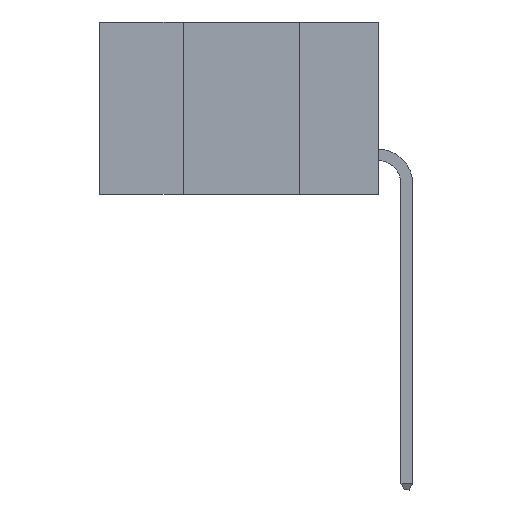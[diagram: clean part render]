
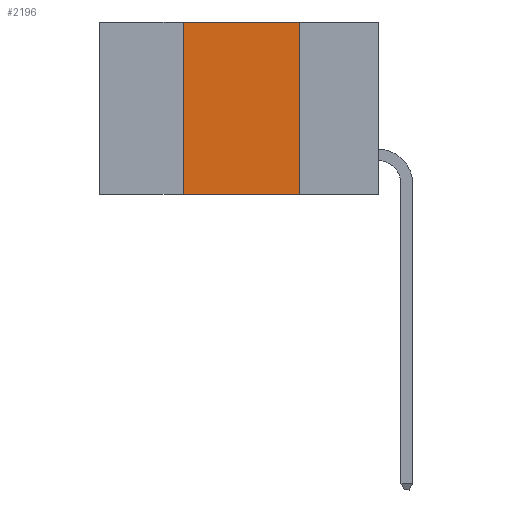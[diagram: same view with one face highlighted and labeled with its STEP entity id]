
A CAD part, left-side view. The second image highlights one B-rep face of the part: STEP entity #2196.
In plain terms, the highlighted planar face has unit normal (-1, 0, 0).
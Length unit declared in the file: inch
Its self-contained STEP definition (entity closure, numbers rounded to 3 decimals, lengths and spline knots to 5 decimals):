
#313 = ORIENTED_EDGE ( 'NONE', *, *, #7847, .T. ) ;
#606 = ORIENTED_EDGE ( 'NONE', *, *, #3129, .F. ) ;
#937 = VECTOR ( 'NONE', #29486, 39.37008 ) ;
#1096 = DIRECTION ( 'NONE',  ( 0., -1., 0. ) ) ;
#1657 = VERTEX_POINT ( 'NONE', #4652 ) ;
#1899 = CARTESIAN_POINT ( 'NONE',  ( 0., 0.6, 0. ) ) ;
#2196 = ADVANCED_FACE ( 'NONE', ( #18134 ), #19116, .F. ) ;
#2372 = LINE ( 'NONE', #12131, #5848 ) ;
#2737 = VERTEX_POINT ( 'NONE', #16178 ) ;
#3129 = EDGE_CURVE ( 'NONE', #22476, #1657, #28222, .T. ) ;
#4652 = CARTESIAN_POINT ( 'NONE',  ( 0., 0.17, 0. ) ) ;
#5111 = DIRECTION ( 'NONE',  ( 0., -1., 0. ) ) ;
#5848 = VECTOR ( 'NONE', #5111, 39.37008 ) ;
#6879 = DIRECTION ( 'NONE',  ( 1., 0., 0. ) ) ;
#7847 = EDGE_CURVE ( 'NONE', #23846, #2737, #2372, .T. ) ;
#7997 = VECTOR ( 'NONE', #1096, 39.37008 ) ;
#10301 = ORIENTED_EDGE ( 'NONE', *, *, #19878, .F. ) ;
#12131 = CARTESIAN_POINT ( 'NONE',  ( 0., 0.6, -0.37 ) ) ;
#12479 = DIRECTION ( 'NONE',  ( 0., 0., 1. ) ) ;
#12748 = LINE ( 'NONE', #29764, #24333 ) ;
#13990 = ORIENTED_EDGE ( 'NONE', *, *, #15978, .F. ) ;
#15978 = EDGE_CURVE ( 'NONE', #1657, #2737, #28776, .T. ) ;
#16178 = CARTESIAN_POINT ( 'NONE',  ( 0., 0.17, -0.37 ) ) ;
#17539 = CARTESIAN_POINT ( 'NONE',  ( 0., 0.17, 0. ) ) ;
#18134 = FACE_OUTER_BOUND ( 'NONE', #24584, .T. ) ;
#19116 = PLANE ( 'NONE',  #29102 ) ;
#19335 = DIRECTION ( 'NONE',  ( 0., 0., -1. ) ) ;
#19878 = EDGE_CURVE ( 'NONE', #23846, #22476, #12748, .T. ) ;
#20315 = CARTESIAN_POINT ( 'NONE',  ( 0., 0.42, -0.37 ) ) ;
#22476 = VERTEX_POINT ( 'NONE', #23418 ) ;
#23418 = CARTESIAN_POINT ( 'NONE',  ( 0., 0.42, 0. ) ) ;
#23846 = VERTEX_POINT ( 'NONE', #20315 ) ;
#24333 = VECTOR ( 'NONE', #12479, 39.37008 ) ;
#24584 = EDGE_LOOP ( 'NONE', ( #13990, #606, #10301, #313 ) ) ;
#26120 = CARTESIAN_POINT ( 'NONE',  ( 0., 0.6, 0. ) ) ;
#28222 = LINE ( 'NONE', #26120, #7997 ) ;
#28776 = LINE ( 'NONE', #17539, #937 ) ;
#29102 = AXIS2_PLACEMENT_3D ( 'NONE', #1899, #6879, #19335 ) ;
#29486 = DIRECTION ( 'NONE',  ( 0., 0., -1. ) ) ;
#29764 = CARTESIAN_POINT ( 'NONE',  ( 0., 0.42, 0. ) ) ;
